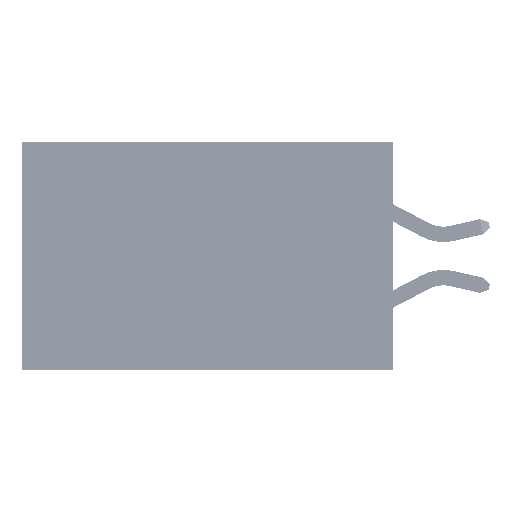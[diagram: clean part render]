
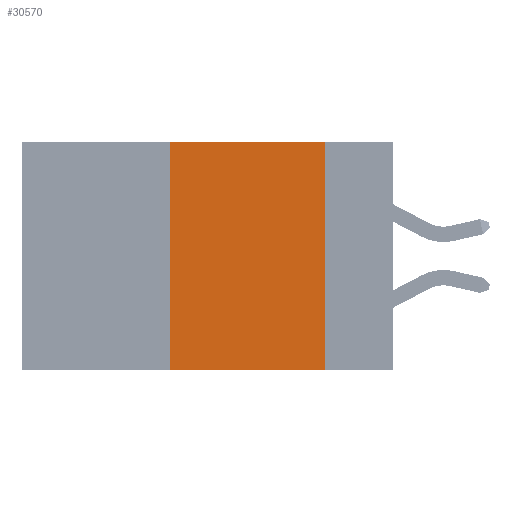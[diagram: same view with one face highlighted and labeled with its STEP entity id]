
A CAD part, left-side view. The second image highlights one B-rep face of the part: STEP entity #30570.
In plain terms, the highlighted planar face has unit normal (-1, 0, 0).
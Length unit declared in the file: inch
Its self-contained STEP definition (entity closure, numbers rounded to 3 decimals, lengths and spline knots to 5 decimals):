
#1942 = VERTEX_POINT ( 'NONE', #24079 ) ;
#3685 = CARTESIAN_POINT ( 'NONE',  ( 0., 0.11, 0. ) ) ;
#4173 = DIRECTION ( 'NONE',  ( 0., 0., -1. ) ) ;
#4586 = VECTOR ( 'NONE', #20161, 39.37008 ) ;
#7535 = CARTESIAN_POINT ( 'NONE',  ( 0., 0.6, 0. ) ) ;
#7903 = LINE ( 'NONE', #10730, #43767 ) ;
#9477 = EDGE_CURVE ( 'NONE', #1942, #10214, #23718, .T. ) ;
#10214 = VERTEX_POINT ( 'NONE', #12719 ) ;
#10730 = CARTESIAN_POINT ( 'NONE',  ( 0., 0.6, -0.37 ) ) ;
#10732 = LINE ( 'NONE', #44380, #44444 ) ;
#12040 = ORIENTED_EDGE ( 'NONE', *, *, #9477, .F. ) ;
#12719 = CARTESIAN_POINT ( 'NONE',  ( 0., 0.36, 0. ) ) ;
#13232 = CARTESIAN_POINT ( 'NONE',  ( 0., 0.11, -0.37 ) ) ;
#14253 = DIRECTION ( 'NONE',  ( 0., -1., 0. ) ) ;
#15226 = AXIS2_PLACEMENT_3D ( 'NONE', #7535, #24884, #4173 ) ;
#19977 = DIRECTION ( 'NONE',  ( 0., -1., 0. ) ) ;
#20161 = DIRECTION ( 'NONE',  ( 0., 0., -1. ) ) ;
#21389 = PLANE ( 'NONE',  #15226 ) ;
#22359 = FACE_OUTER_BOUND ( 'NONE', #36639, .T. ) ;
#23718 = LINE ( 'NONE', #38597, #33078 ) ;
#24079 = CARTESIAN_POINT ( 'NONE',  ( 0., 0.36, -0.37 ) ) ;
#24817 = EDGE_CURVE ( 'NONE', #1942, #31384, #7903, .T. ) ;
#24884 = DIRECTION ( 'NONE',  ( 1., 0., 0. ) ) ;
#25307 = EDGE_CURVE ( 'NONE', #37463, #31384, #32324, .T. ) ;
#26873 = ORIENTED_EDGE ( 'NONE', *, *, #24817, .T. ) ;
#30570 = ADVANCED_FACE ( 'NONE', ( #22359 ), #21389, .F. ) ;
#31384 = VERTEX_POINT ( 'NONE', #13232 ) ;
#32324 = LINE ( 'NONE', #34102, #4586 ) ;
#33078 = VECTOR ( 'NONE', #41458, 39.37008 ) ;
#33224 = ORIENTED_EDGE ( 'NONE', *, *, #25307, .F. ) ;
#34102 = CARTESIAN_POINT ( 'NONE',  ( 0., 0.11, 0. ) ) ;
#34979 = ORIENTED_EDGE ( 'NONE', *, *, #44702, .F. ) ;
#36639 = EDGE_LOOP ( 'NONE', ( #33224, #34979, #12040, #26873 ) ) ;
#37463 = VERTEX_POINT ( 'NONE', #3685 ) ;
#38597 = CARTESIAN_POINT ( 'NONE',  ( 0., 0.36, 0. ) ) ;
#41458 = DIRECTION ( 'NONE',  ( 0., 0., 1. ) ) ;
#43767 = VECTOR ( 'NONE', #14253, 39.37008 ) ;
#44380 = CARTESIAN_POINT ( 'NONE',  ( 0., 0.6, 0. ) ) ;
#44444 = VECTOR ( 'NONE', #19977, 39.37008 ) ;
#44702 = EDGE_CURVE ( 'NONE', #10214, #37463, #10732, .T. ) ;
